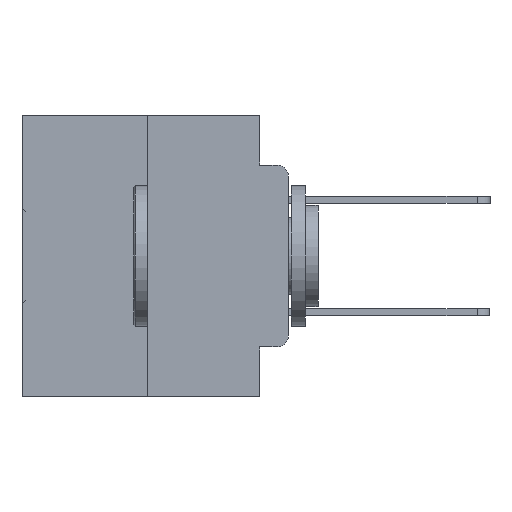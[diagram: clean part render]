
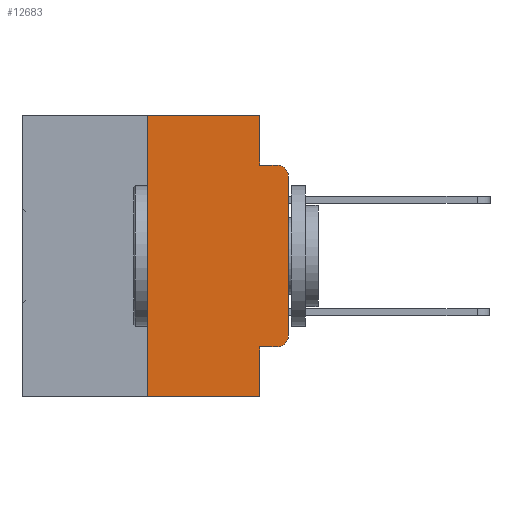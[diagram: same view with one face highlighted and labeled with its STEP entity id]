
A CAD part, left-side view. The second image highlights one B-rep face of the part: STEP entity #12683.
In plain terms, the highlighted planar face has unit normal (-1, 0, 0).
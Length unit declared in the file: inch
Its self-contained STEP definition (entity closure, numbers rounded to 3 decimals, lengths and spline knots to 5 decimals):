
#847 = EDGE_CURVE ( 'NONE', #5042, #32038, #33483, .T. ) ;
#1104 = VERTEX_POINT ( 'NONE', #7027 ) ;
#1411 = DIRECTION ( 'NONE',  ( 0., 0., -1. ) ) ;
#1427 = VERTEX_POINT ( 'NONE', #11473 ) ;
#1572 = VECTOR ( 'NONE', #24050, 39.37008 ) ;
#1859 = LINE ( 'NONE', #21963, #2692 ) ;
#2692 = VECTOR ( 'NONE', #6112, 39.37008 ) ;
#2741 = DIRECTION ( 'NONE',  ( 0., 0., -1. ) ) ;
#3140 = EDGE_CURVE ( 'NONE', #17985, #1104, #22703, .T. ) ;
#3465 = CARTESIAN_POINT ( 'NONE',  ( 0., 0., 0. ) ) ;
#3772 = EDGE_CURVE ( 'NONE', #6752, #1427, #10225, .T. ) ;
#4305 = CIRCLE ( 'NONE', #22446, 0.02 ) ;
#4603 = CARTESIAN_POINT ( 'NONE',  ( 0., 0.02, -0.0885 ) ) ;
#5042 = VERTEX_POINT ( 'NONE', #29237 ) ;
#5371 = EDGE_CURVE ( 'NONE', #1104, #26791, #20478, .T. ) ;
#5440 = VECTOR ( 'NONE', #25488, 39.37008 ) ;
#6112 = DIRECTION ( 'NONE',  ( 0., -1., 0. ) ) ;
#6752 = VERTEX_POINT ( 'NONE', #10147 ) ;
#6869 = EDGE_CURVE ( 'NONE', #32038, #13521, #4305, .T. ) ;
#7027 = CARTESIAN_POINT ( 'NONE',  ( 0., 0.051, 0. ) ) ;
#7091 = ORIENTED_EDGE ( 'NONE', *, *, #31990, .F. ) ;
#8456 = LINE ( 'NONE', #19892, #33215 ) ;
#8756 = FACE_OUTER_BOUND ( 'NONE', #16837, .T. ) ;
#9194 = EDGE_CURVE ( 'NONE', #1427, #5042, #24743, .T. ) ;
#9328 = DIRECTION ( 'NONE',  ( 0., 0., -1. ) ) ;
#10147 = CARTESIAN_POINT ( 'NONE',  ( 0., 0.051, -0.4115 ) ) ;
#10225 = LINE ( 'NONE', #24101, #28872 ) ;
#10693 = DIRECTION ( 'NONE',  ( -1., 0., 0. ) ) ;
#11473 = CARTESIAN_POINT ( 'NONE',  ( 0., 0.02, -0.4115 ) ) ;
#12683 = ADVANCED_FACE ( 'NONE', ( #8756 ), #26323, .F. ) ;
#12705 = ORIENTED_EDGE ( 'NONE', *, *, #5371, .F. ) ;
#12838 = EDGE_CURVE ( 'NONE', #26791, #13521, #22432, .T. ) ;
#13408 = VECTOR ( 'NONE', #9328, 39.37008 ) ;
#13521 = VERTEX_POINT ( 'NONE', #4603 ) ;
#13930 = CARTESIAN_POINT ( 'NONE',  ( 0., 0.051, -0.0885 ) ) ;
#13933 = DIRECTION ( 'NONE',  ( 0., 0., 1. ) ) ;
#14705 = CARTESIAN_POINT ( 'NONE',  ( 0., 0.051, -0.0885 ) ) ;
#15688 = DIRECTION ( 'NONE',  ( -1., 0., 0. ) ) ;
#16472 = EDGE_CURVE ( 'NONE', #20781, #28588, #1859, .T. ) ;
#16837 = EDGE_LOOP ( 'NONE', ( #27203, #20574, #33345, #12705, #20231, #27752, #19043, #7091, #33885, #22722 ) ) ;
#17050 = CARTESIAN_POINT ( 'NONE',  ( 0., 0.051, 0. ) ) ;
#17110 = AXIS2_PLACEMENT_3D ( 'NONE', #31476, #15688, #34072 ) ;
#17985 = VERTEX_POINT ( 'NONE', #20105 ) ;
#18445 = EDGE_CURVE ( 'NONE', #20781, #17985, #32614, .T. ) ;
#18550 = DIRECTION ( 'NONE',  ( 1., 0., 0. ) ) ;
#18578 = CARTESIAN_POINT ( 'NONE',  ( 0., 0.051, -0.5 ) ) ;
#19043 = ORIENTED_EDGE ( 'NONE', *, *, #16472, .T. ) ;
#19892 = CARTESIAN_POINT ( 'NONE',  ( 0., 0.051, 0. ) ) ;
#20105 = CARTESIAN_POINT ( 'NONE',  ( 0., 0.25, 0. ) ) ;
#20231 = ORIENTED_EDGE ( 'NONE', *, *, #3140, .F. ) ;
#20478 = LINE ( 'NONE', #17050, #13408 ) ;
#20574 = ORIENTED_EDGE ( 'NONE', *, *, #6869, .T. ) ;
#20781 = VERTEX_POINT ( 'NONE', #26227 ) ;
#21963 = CARTESIAN_POINT ( 'NONE',  ( 0., 0.473, -0.5 ) ) ;
#22081 = CARTESIAN_POINT ( 'NONE',  ( 0., 0.473, 0. ) ) ;
#22432 = LINE ( 'NONE', #13930, #29423 ) ;
#22446 = AXIS2_PLACEMENT_3D ( 'NONE', #26588, #10693, #29241 ) ;
#22703 = LINE ( 'NONE', #27887, #1572 ) ;
#22722 = ORIENTED_EDGE ( 'NONE', *, *, #9194, .T. ) ;
#23895 = AXIS2_PLACEMENT_3D ( 'NONE', #22081, #18550, #2741 ) ;
#24050 = DIRECTION ( 'NONE',  ( 0., -1., 0. ) ) ;
#24101 = CARTESIAN_POINT ( 'NONE',  ( 0., 0.051, -0.4115 ) ) ;
#24743 = CIRCLE ( 'NONE', #17110, 0.02 ) ;
#25316 = DIRECTION ( 'NONE',  ( 0., -1., 0. ) ) ;
#25488 = DIRECTION ( 'NONE',  ( 0., 0., 1. ) ) ;
#26227 = CARTESIAN_POINT ( 'NONE',  ( 0., 0.25, -0.5 ) ) ;
#26323 = PLANE ( 'NONE',  #23895 ) ;
#26588 = CARTESIAN_POINT ( 'NONE',  ( 0., 0.02, -0.1085 ) ) ;
#26791 = VERTEX_POINT ( 'NONE', #14705 ) ;
#27203 = ORIENTED_EDGE ( 'NONE', *, *, #847, .T. ) ;
#27752 = ORIENTED_EDGE ( 'NONE', *, *, #18445, .F. ) ;
#27887 = CARTESIAN_POINT ( 'NONE',  ( 0., 0.473, 0. ) ) ;
#28588 = VERTEX_POINT ( 'NONE', #18578 ) ;
#28872 = VECTOR ( 'NONE', #25316, 39.37008 ) ;
#29237 = CARTESIAN_POINT ( 'NONE',  ( 0., 0., -0.3915 ) ) ;
#29241 = DIRECTION ( 'NONE',  ( 0., 0., -1. ) ) ;
#29423 = VECTOR ( 'NONE', #32375, 39.37008 ) ;
#30648 = CARTESIAN_POINT ( 'NONE',  ( 0., 0., -0.1085 ) ) ;
#31476 = CARTESIAN_POINT ( 'NONE',  ( 0., 0.02, -0.3915 ) ) ;
#31990 = EDGE_CURVE ( 'NONE', #6752, #28588, #8456, .T. ) ;
#32038 = VERTEX_POINT ( 'NONE', #30648 ) ;
#32375 = DIRECTION ( 'NONE',  ( 0., -1., 0. ) ) ;
#32377 = CARTESIAN_POINT ( 'NONE',  ( 0., 0.25, 0. ) ) ;
#32614 = LINE ( 'NONE', #32377, #33435 ) ;
#33215 = VECTOR ( 'NONE', #1411, 39.37008 ) ;
#33345 = ORIENTED_EDGE ( 'NONE', *, *, #12838, .F. ) ;
#33435 = VECTOR ( 'NONE', #13933, 39.37008 ) ;
#33483 = LINE ( 'NONE', #3465, #5440 ) ;
#33885 = ORIENTED_EDGE ( 'NONE', *, *, #3772, .T. ) ;
#34072 = DIRECTION ( 'NONE',  ( 0., 0., -1. ) ) ;
